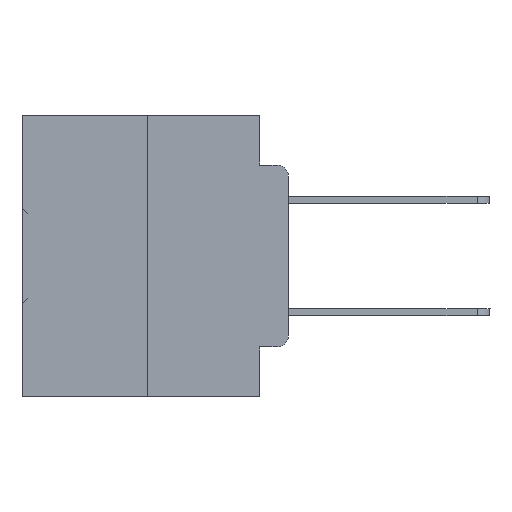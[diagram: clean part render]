
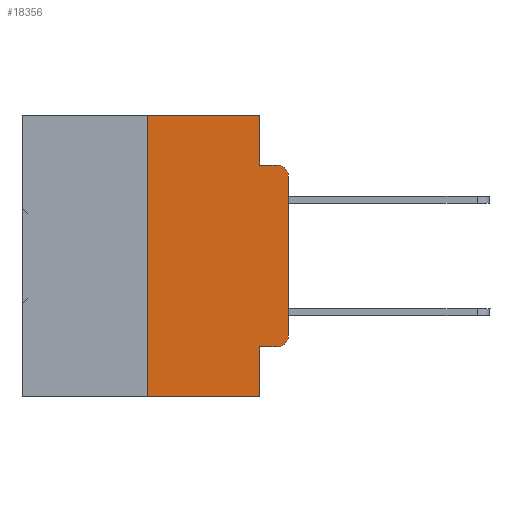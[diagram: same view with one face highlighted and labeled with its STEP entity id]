
A CAD part, left-side view. The second image highlights one B-rep face of the part: STEP entity #18356.
In plain terms, the highlighted planar face has unit normal (-1, 0, 0).
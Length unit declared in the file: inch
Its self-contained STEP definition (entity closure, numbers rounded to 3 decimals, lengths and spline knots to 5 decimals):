
#237 = VERTEX_POINT ( 'NONE', #13679 ) ;
#656 = CARTESIAN_POINT ( 'NONE',  ( 0., 0.051, -0.4115 ) ) ;
#745 = CARTESIAN_POINT ( 'NONE',  ( 0., 0.051, -0.5 ) ) ;
#1296 = DIRECTION ( 'NONE',  ( 0., 0., -1. ) ) ;
#2034 = DIRECTION ( 'NONE',  ( 1., 0., 0. ) ) ;
#2336 = VECTOR ( 'NONE', #12598, 39.37008 ) ;
#2394 = DIRECTION ( 'NONE',  ( 0., 0., 1. ) ) ;
#2715 = LINE ( 'NONE', #28705, #19001 ) ;
#4331 = LINE ( 'NONE', #26679, #16881 ) ;
#4703 = CARTESIAN_POINT ( 'NONE',  ( 0., 0., -0.3915 ) ) ;
#4905 = PLANE ( 'NONE',  #27814 ) ;
#5128 = CARTESIAN_POINT ( 'NONE',  ( 0., 0.02, -0.0885 ) ) ;
#6106 = DIRECTION ( 'NONE',  ( 0., 0., 1. ) ) ;
#6657 = CARTESIAN_POINT ( 'NONE',  ( 0., 0., 0. ) ) ;
#6801 = EDGE_CURVE ( 'NONE', #36575, #237, #30149, .T. ) ;
#7029 = ORIENTED_EDGE ( 'NONE', *, *, #7640, .T. ) ;
#7197 = VECTOR ( 'NONE', #11211, 39.37008 ) ;
#7230 = ORIENTED_EDGE ( 'NONE', *, *, #27120, .F. ) ;
#7414 = ORIENTED_EDGE ( 'NONE', *, *, #23926, .F. ) ;
#7640 = EDGE_CURVE ( 'NONE', #29885, #28030, #14761, .T. ) ;
#7800 = DIRECTION ( 'NONE',  ( -1., 0., 0. ) ) ;
#8409 = EDGE_CURVE ( 'NONE', #14039, #36045, #2715, .T. ) ;
#8834 = CARTESIAN_POINT ( 'NONE',  ( 0., 0.473, 0. ) ) ;
#9300 = DIRECTION ( 'NONE',  ( 0., 0., -1. ) ) ;
#9783 = VECTOR ( 'NONE', #2394, 39.37008 ) ;
#10086 = VERTEX_POINT ( 'NONE', #33045 ) ;
#10159 = ORIENTED_EDGE ( 'NONE', *, *, #18120, .F. ) ;
#10161 = VERTEX_POINT ( 'NONE', #745 ) ;
#10287 = CARTESIAN_POINT ( 'NONE',  ( 0., 0.473, 0. ) ) ;
#10649 = LINE ( 'NONE', #22643, #9783 ) ;
#11211 = DIRECTION ( 'NONE',  ( 0., 0., -1. ) ) ;
#11904 = CARTESIAN_POINT ( 'NONE',  ( 0., 0.051, -0.4115 ) ) ;
#12154 = CARTESIAN_POINT ( 'NONE',  ( 0., 0.02, -0.3915 ) ) ;
#12366 = CARTESIAN_POINT ( 'NONE',  ( 0., 0.051, -0.0885 ) ) ;
#12598 = DIRECTION ( 'NONE',  ( 0., -1., 0. ) ) ;
#12980 = LINE ( 'NONE', #18876, #2336 ) ;
#13038 = ORIENTED_EDGE ( 'NONE', *, *, #27924, .T. ) ;
#13679 = CARTESIAN_POINT ( 'NONE',  ( 0., 0., -0.1085 ) ) ;
#13723 = DIRECTION ( 'NONE',  ( 0., 0., -1. ) ) ;
#13899 = ORIENTED_EDGE ( 'NONE', *, *, #18497, .T. ) ;
#14039 = VERTEX_POINT ( 'NONE', #12366 ) ;
#14404 = ORIENTED_EDGE ( 'NONE', *, *, #29861, .F. ) ;
#14717 = VECTOR ( 'NONE', #35007, 39.37008 ) ;
#14761 = LINE ( 'NONE', #11904, #24449 ) ;
#16808 = DIRECTION ( 'NONE',  ( 0., 0., -1. ) ) ;
#16881 = VECTOR ( 'NONE', #1296, 39.37008 ) ;
#16908 = AXIS2_PLACEMENT_3D ( 'NONE', #12154, #23765, #9300 ) ;
#17075 = CIRCLE ( 'NONE', #22522, 0.02 ) ;
#18120 = EDGE_CURVE ( 'NONE', #10086, #14039, #4331, .T. ) ;
#18356 = ADVANCED_FACE ( 'NONE', ( #25330 ), #4905, .F. ) ;
#18497 = EDGE_CURVE ( 'NONE', #28030, #36575, #22967, .T. ) ;
#18876 = CARTESIAN_POINT ( 'NONE',  ( 0., 0.473, -0.5 ) ) ;
#19001 = VECTOR ( 'NONE', #20090, 39.37008 ) ;
#19406 = VECTOR ( 'NONE', #6106, 39.37008 ) ;
#20090 = DIRECTION ( 'NONE',  ( 0., -1., 0. ) ) ;
#20661 = EDGE_CURVE ( 'NONE', #237, #36045, #17075, .T. ) ;
#22522 = AXIS2_PLACEMENT_3D ( 'NONE', #26099, #7800, #16808 ) ;
#22600 = EDGE_LOOP ( 'NONE', ( #23198, #24071, #33399, #10159, #7414, #14404, #13038, #7230, #7029, #13899 ) ) ;
#22643 = CARTESIAN_POINT ( 'NONE',  ( 0., 0.25, 0. ) ) ;
#22967 = CIRCLE ( 'NONE', #16908, 0.02 ) ;
#23153 = CARTESIAN_POINT ( 'NONE',  ( 0., 0.25, 0. ) ) ;
#23198 = ORIENTED_EDGE ( 'NONE', *, *, #6801, .T. ) ;
#23487 = LINE ( 'NONE', #8834, #14717 ) ;
#23765 = DIRECTION ( 'NONE',  ( -1., 0., 0. ) ) ;
#23908 = CARTESIAN_POINT ( 'NONE',  ( 0., 0.25, -0.5 ) ) ;
#23926 = EDGE_CURVE ( 'NONE', #36773, #10086, #23487, .T. ) ;
#24071 = ORIENTED_EDGE ( 'NONE', *, *, #20661, .T. ) ;
#24449 = VECTOR ( 'NONE', #35210, 39.37008 ) ;
#25301 = LINE ( 'NONE', #33927, #7197 ) ;
#25330 = FACE_OUTER_BOUND ( 'NONE', #22600, .T. ) ;
#26099 = CARTESIAN_POINT ( 'NONE',  ( 0., 0.02, -0.1085 ) ) ;
#26679 = CARTESIAN_POINT ( 'NONE',  ( 0., 0.051, 0. ) ) ;
#27120 = EDGE_CURVE ( 'NONE', #29885, #10161, #25301, .T. ) ;
#27814 = AXIS2_PLACEMENT_3D ( 'NONE', #10287, #2034, #13723 ) ;
#27924 = EDGE_CURVE ( 'NONE', #34718, #10161, #12980, .T. ) ;
#28030 = VERTEX_POINT ( 'NONE', #37420 ) ;
#28705 = CARTESIAN_POINT ( 'NONE',  ( 0., 0.051, -0.0885 ) ) ;
#29861 = EDGE_CURVE ( 'NONE', #34718, #36773, #10649, .T. ) ;
#29885 = VERTEX_POINT ( 'NONE', #656 ) ;
#30149 = LINE ( 'NONE', #6657, #19406 ) ;
#33045 = CARTESIAN_POINT ( 'NONE',  ( 0., 0.051, 0. ) ) ;
#33399 = ORIENTED_EDGE ( 'NONE', *, *, #8409, .F. ) ;
#33927 = CARTESIAN_POINT ( 'NONE',  ( 0., 0.051, 0. ) ) ;
#34718 = VERTEX_POINT ( 'NONE', #23908 ) ;
#35007 = DIRECTION ( 'NONE',  ( 0., -1., 0. ) ) ;
#35210 = DIRECTION ( 'NONE',  ( 0., -1., 0. ) ) ;
#36045 = VERTEX_POINT ( 'NONE', #5128 ) ;
#36575 = VERTEX_POINT ( 'NONE', #4703 ) ;
#36773 = VERTEX_POINT ( 'NONE', #23153 ) ;
#37420 = CARTESIAN_POINT ( 'NONE',  ( 0., 0.02, -0.4115 ) ) ;
